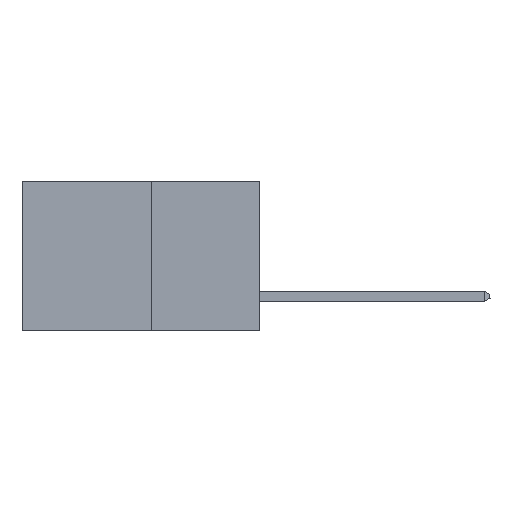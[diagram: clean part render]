
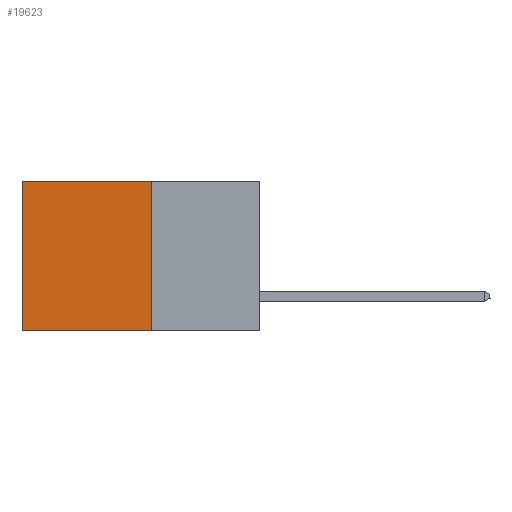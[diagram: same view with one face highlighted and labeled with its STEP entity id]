
A CAD part, left-side view. The second image highlights one B-rep face of the part: STEP entity #19623.
In plain terms, the highlighted planar face has unit normal (-1, 0, 0).
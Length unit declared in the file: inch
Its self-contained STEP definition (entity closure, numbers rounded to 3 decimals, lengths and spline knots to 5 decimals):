
#334 = FACE_OUTER_BOUND ( 'NONE', #5143, .T. ) ;
#928 = CARTESIAN_POINT ( 'NONE',  ( 0.277, 0.27, -0.37 ) ) ;
#2399 = EDGE_CURVE ( 'NONE', #14191, #14652, #5077, .T. ) ;
#3017 = DIRECTION ( 'NONE',  ( 1., 0., 0. ) ) ;
#4287 = VECTOR ( 'NONE', #17587, 39.37008 ) ;
#5077 = LINE ( 'NONE', #12240, #8637 ) ;
#5143 = EDGE_LOOP ( 'NONE', ( #13141, #14240, #9816, #6621 ) ) ;
#5663 = EDGE_CURVE ( 'NONE', #11500, #14191, #9773, .T. ) ;
#6548 = CARTESIAN_POINT ( 'NONE',  ( 0.277, 0.59, -0.37 ) ) ;
#6621 = ORIENTED_EDGE ( 'NONE', *, *, #13948, .T. ) ;
#7776 = VECTOR ( 'NONE', #7967, 39.37008 ) ;
#7967 = DIRECTION ( 'NONE',  ( 0., 1., 0. ) ) ;
#8637 = VECTOR ( 'NONE', #19305, 39.37008 ) ;
#8810 = LINE ( 'NONE', #11395, #4287 ) ;
#9042 = PLANE ( 'NONE',  #14540 ) ;
#9773 = LINE ( 'NONE', #13902, #10256 ) ;
#9816 = ORIENTED_EDGE ( 'NONE', *, *, #5663, .F. ) ;
#10256 = VECTOR ( 'NONE', #13842, 39.37008 ) ;
#11395 = CARTESIAN_POINT ( 'NONE',  ( 0.277, 0.59, -0.37 ) ) ;
#11500 = VERTEX_POINT ( 'NONE', #18841 ) ;
#12169 = CARTESIAN_POINT ( 'NONE',  ( 0.277, 0.27, -0.37 ) ) ;
#12240 = CARTESIAN_POINT ( 'NONE',  ( 0.277, 0.27, -0.37 ) ) ;
#13141 = ORIENTED_EDGE ( 'NONE', *, *, #16016, .T. ) ;
#13522 = CARTESIAN_POINT ( 'NONE',  ( 0.277, 0.59, 0. ) ) ;
#13700 = DIRECTION ( 'NONE',  ( 0., 0., -1. ) ) ;
#13842 = DIRECTION ( 'NONE',  ( 0., 0., -1. ) ) ;
#13902 = CARTESIAN_POINT ( 'NONE',  ( 0.277, 0.27, -0.37 ) ) ;
#13948 = EDGE_CURVE ( 'NONE', #11500, #18532, #15969, .T. ) ;
#14191 = VERTEX_POINT ( 'NONE', #928 ) ;
#14240 = ORIENTED_EDGE ( 'NONE', *, *, #2399, .F. ) ;
#14540 = AXIS2_PLACEMENT_3D ( 'NONE', #12169, #3017, #13700 ) ;
#14652 = VERTEX_POINT ( 'NONE', #6548 ) ;
#15969 = LINE ( 'NONE', #18707, #7776 ) ;
#16016 = EDGE_CURVE ( 'NONE', #18532, #14652, #8810, .T. ) ;
#17587 = DIRECTION ( 'NONE',  ( 0., 0., -1. ) ) ;
#18532 = VERTEX_POINT ( 'NONE', #13522 ) ;
#18707 = CARTESIAN_POINT ( 'NONE',  ( 0.277, 0.27, 0. ) ) ;
#18841 = CARTESIAN_POINT ( 'NONE',  ( 0.277, 0.27, 0. ) ) ;
#19305 = DIRECTION ( 'NONE',  ( 0., 1., 0. ) ) ;
#19623 = ADVANCED_FACE ( 'NONE', ( #334 ), #9042, .F. ) ;
